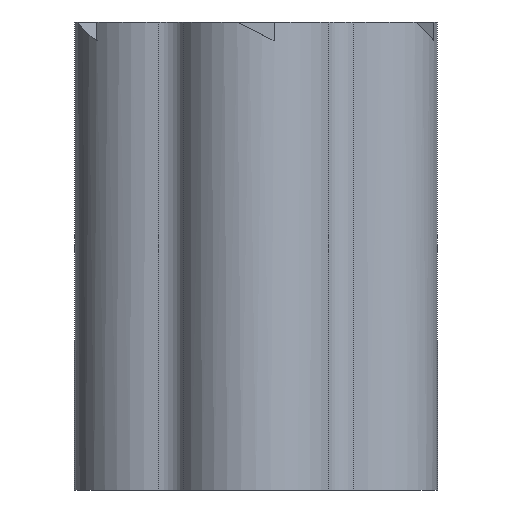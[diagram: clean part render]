
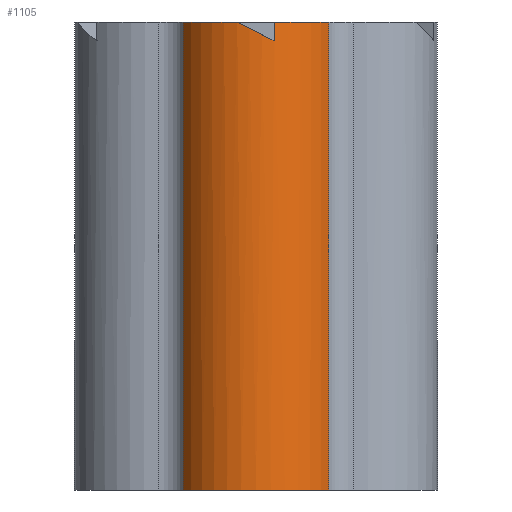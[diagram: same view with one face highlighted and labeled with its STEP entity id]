
A CAD part, front view. The second image highlights one B-rep face of the part: STEP entity #1105.
In plain terms, the highlighted cylindrical face has radius 9 mm (diameter 18 mm), a partial arc.
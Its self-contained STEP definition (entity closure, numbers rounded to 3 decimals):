
#448=CARTESIAN_POINT('',(-2.,-32.775,50.0));
#449=VERTEX_POINT('',#448);
#456=CARTESIAN_POINT('',(1.925,-32.792,48.0));
#457=VERTEX_POINT('',#456);
#458=CARTESIAN_POINT('',(0.0,-24.,48.981));
#459=DIRECTION('',(0.454,0.0,0.891));
#460=DIRECTION('',(0.891,0.0,-0.454));
#461=AXIS2_PLACEMENT_3D('',#458,#459,#460);
#462=ELLIPSE('',#461,10.101,9.0);
#463=EDGE_CURVE('',#449,#457,#462,.T.);
#480=CARTESIAN_POINT('',(2.,-32.775,48.0));
#481=VERTEX_POINT('',#480);
#482=CARTESIAN_POINT('',(0.0,-24.,48.0));
#483=DIRECTION('',(0.0,0.0,-1.0));
#484=DIRECTION('',(0.866,0.5,0.0));
#485=AXIS2_PLACEMENT_3D('',#482,#483,#484);
#486=CIRCLE('',#485,9.);
#487=EDGE_CURVE('',#481,#457,#486,.T.);
#1013=CARTESIAN_POINT('',(2.,-32.775,50.0));
#1014=VERTEX_POINT('',#1013);
#1028=CARTESIAN_POINT('',(2.,-32.775,50.0));
#1029=DIRECTION('',(0.0,0.0,-1.0));
#1030=VECTOR('',#1029,2.0);
#1031=LINE('',#1028,#1030);
#1032=EDGE_CURVE('',#1014,#481,#1031,.T.);
#1054=CARTESIAN_POINT('',(0.0,-24.,0.0));
#1055=DIRECTION('',(0.0,0.0,1.0));
#1056=DIRECTION('',(0.866,0.5,0.0));
#1057=AXIS2_PLACEMENT_3D('',#1054,#1055,#1056);
#1058=CYLINDRICAL_SURFACE('',#1057,9.0);
#1059=ORIENTED_EDGE('',*,*,#1032,.T.);
#1060=ORIENTED_EDGE('',*,*,#487,.T.);
#1061=ORIENTED_EDGE('',*,*,#463,.F.);
#1062=CARTESIAN_POINT('',(-7.794,-28.5,50.0));
#1063=VERTEX_POINT('',#1062);
#1064=CARTESIAN_POINT('',(0.0,-24.,50.0));
#1065=DIRECTION('',(0.0,0.0,1.0));
#1066=DIRECTION('',(0.866,0.5,0.0));
#1067=AXIS2_PLACEMENT_3D('',#1064,#1065,#1066);
#1068=CIRCLE('',#1067,9.);
#1069=EDGE_CURVE('',#1063,#449,#1068,.T.);
#1070=ORIENTED_EDGE('',*,*,#1069,.F.);
#1071=CARTESIAN_POINT('',(-7.794,-28.5,0.0));
#1072=VERTEX_POINT('',#1071);
#1073=CARTESIAN_POINT('',(-7.794,-28.5,0.0));
#1074=DIRECTION('',(0.0,0.0,1.0));
#1075=VECTOR('',#1074,50.0);
#1076=LINE('',#1073,#1075);
#1077=EDGE_CURVE('',#1072,#1063,#1076,.T.);
#1078=ORIENTED_EDGE('',*,*,#1077,.F.);
#1079=CARTESIAN_POINT('',(7.794,-28.5,0.0));
#1080=VERTEX_POINT('',#1079);
#1081=CARTESIAN_POINT('',(0.0,-24.,0.0));
#1082=DIRECTION('',(0.0,0.0,-1.0));
#1083=DIRECTION('',(0.866,0.5,0.0));
#1084=AXIS2_PLACEMENT_3D('',#1081,#1082,#1083);
#1085=CIRCLE('',#1084,9.);
#1086=EDGE_CURVE('',#1080,#1072,#1085,.T.);
#1087=ORIENTED_EDGE('',*,*,#1086,.F.);
#1088=CARTESIAN_POINT('',(7.794,-28.5,50.0));
#1089=VERTEX_POINT('',#1088);
#1090=CARTESIAN_POINT('',(7.794,-28.5,0.0));
#1091=DIRECTION('',(0.0,0.0,1.0));
#1092=VECTOR('',#1091,50.0);
#1093=LINE('',#1090,#1092);
#1094=EDGE_CURVE('',#1080,#1089,#1093,.T.);
#1095=ORIENTED_EDGE('',*,*,#1094,.T.);
#1096=CARTESIAN_POINT('',(0.0,-24.,50.0));
#1097=DIRECTION('',(0.0,0.0,1.0));
#1098=DIRECTION('',(0.866,0.5,0.0));
#1099=AXIS2_PLACEMENT_3D('',#1096,#1097,#1098);
#1100=CIRCLE('',#1099,9.);
#1101=EDGE_CURVE('',#1014,#1089,#1100,.T.);
#1102=ORIENTED_EDGE('',*,*,#1101,.F.);
#1103=EDGE_LOOP('',(#1059,#1060,#1061,#1070,#1078,#1087,#1095,#1102));
#1104=FACE_OUTER_BOUND('',#1103,.T.);
#1105=ADVANCED_FACE('',(#1104),#1058,.T.);
